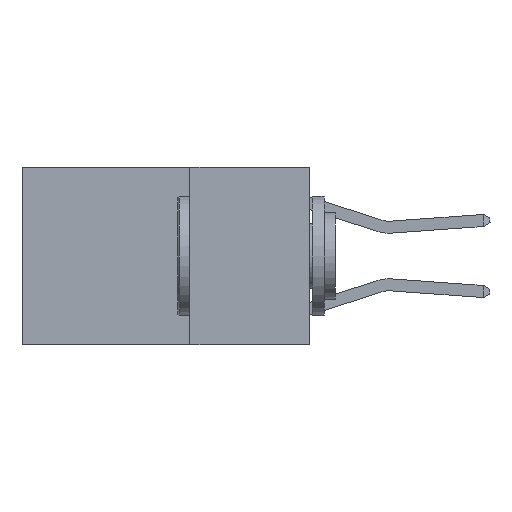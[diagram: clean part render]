
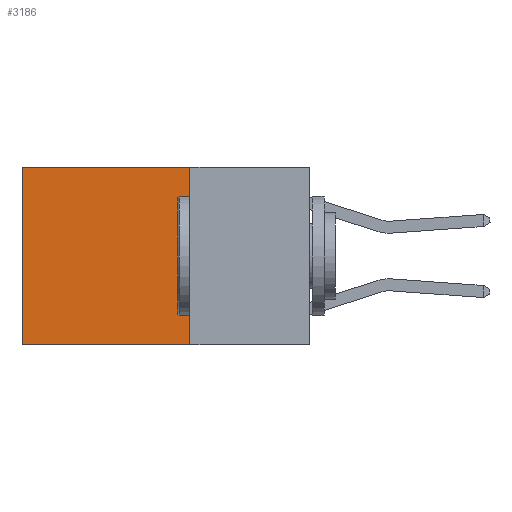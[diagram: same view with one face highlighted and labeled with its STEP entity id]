
A CAD part, left-side view. The second image highlights one B-rep face of the part: STEP entity #3186.
In plain terms, the highlighted planar face has unit normal (-1, 0, 0).
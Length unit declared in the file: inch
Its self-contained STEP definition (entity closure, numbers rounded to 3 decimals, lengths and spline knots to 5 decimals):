
#4 = VECTOR ( 'NONE', #11823, 39.37008 ) ;
#313 = VERTEX_POINT ( 'NONE', #4484 ) ;
#1489 = CARTESIAN_POINT ( 'NONE',  ( 0.2625, 0.25, 0. ) ) ;
#1791 = VERTEX_POINT ( 'NONE', #12470 ) ;
#1855 = CARTESIAN_POINT ( 'NONE',  ( 0.2625, 0.25, -0.37 ) ) ;
#2260 = ORIENTED_EDGE ( 'NONE', *, *, #4013, .T. ) ;
#2300 = DIRECTION ( 'NONE',  ( 1., 0., 0. ) ) ;
#2871 = EDGE_CURVE ( 'NONE', #1791, #7134, #14022, .T. ) ;
#2988 = ORIENTED_EDGE ( 'NONE', *, *, #11942, .F. ) ;
#3035 = DIRECTION ( 'NONE',  ( 0., 1., 0. ) ) ;
#3186 = ADVANCED_FACE ( 'NONE', ( #10870 ), #8251, .F. ) ;
#3468 = LINE ( 'NONE', #1855, #12142 ) ;
#4013 = EDGE_CURVE ( 'NONE', #1791, #313, #4695, .T. ) ;
#4484 = CARTESIAN_POINT ( 'NONE',  ( 0.2625, 0.6, 0. ) ) ;
#4695 = LINE ( 'NONE', #1489, #11013 ) ;
#4753 = EDGE_CURVE ( 'NONE', #313, #14495, #9479, .T. ) ;
#5178 = CARTESIAN_POINT ( 'NONE',  ( 0.2625, 0.6, 0. ) ) ;
#5519 = CARTESIAN_POINT ( 'NONE',  ( 0.2625, 0.6, -0.37 ) ) ;
#6377 = EDGE_LOOP ( 'NONE', ( #14476, #2988, #8904, #2260 ) ) ;
#7134 = VERTEX_POINT ( 'NONE', #9211 ) ;
#7485 = DIRECTION ( 'NONE',  ( 0., 0., -1. ) ) ;
#8251 = PLANE ( 'NONE',  #14239 ) ;
#8598 = DIRECTION ( 'NONE',  ( 0., 1., 0. ) ) ;
#8904 = ORIENTED_EDGE ( 'NONE', *, *, #2871, .F. ) ;
#9211 = CARTESIAN_POINT ( 'NONE',  ( 0.2625, 0.25, -0.37 ) ) ;
#9479 = LINE ( 'NONE', #5178, #4 ) ;
#10353 = CARTESIAN_POINT ( 'NONE',  ( 0.2625, 0.25, 0. ) ) ;
#10405 = DIRECTION ( 'NONE',  ( 0., 0., -1. ) ) ;
#10870 = FACE_OUTER_BOUND ( 'NONE', #6377, .T. ) ;
#11013 = VECTOR ( 'NONE', #8598, 39.37008 ) ;
#11211 = VECTOR ( 'NONE', #7485, 39.37008 ) ;
#11764 = CARTESIAN_POINT ( 'NONE',  ( 0.2625, 0.25, 0. ) ) ;
#11823 = DIRECTION ( 'NONE',  ( 0., 0., -1. ) ) ;
#11942 = EDGE_CURVE ( 'NONE', #7134, #14495, #3468, .T. ) ;
#12142 = VECTOR ( 'NONE', #3035, 39.37008 ) ;
#12470 = CARTESIAN_POINT ( 'NONE',  ( 0.2625, 0.25, 0. ) ) ;
#14022 = LINE ( 'NONE', #11764, #11211 ) ;
#14239 = AXIS2_PLACEMENT_3D ( 'NONE', #10353, #2300, #10405 ) ;
#14476 = ORIENTED_EDGE ( 'NONE', *, *, #4753, .T. ) ;
#14495 = VERTEX_POINT ( 'NONE', #5519 ) ;
